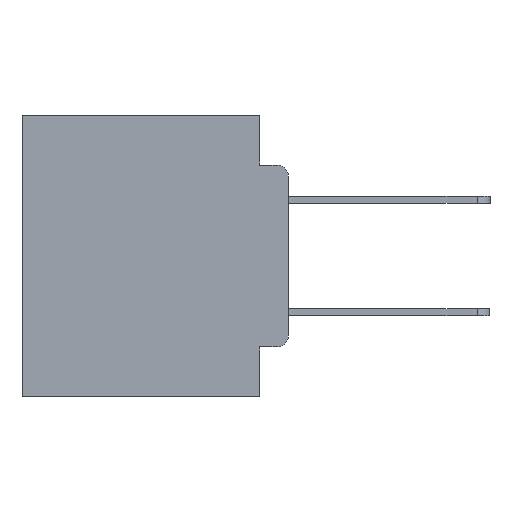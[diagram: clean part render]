
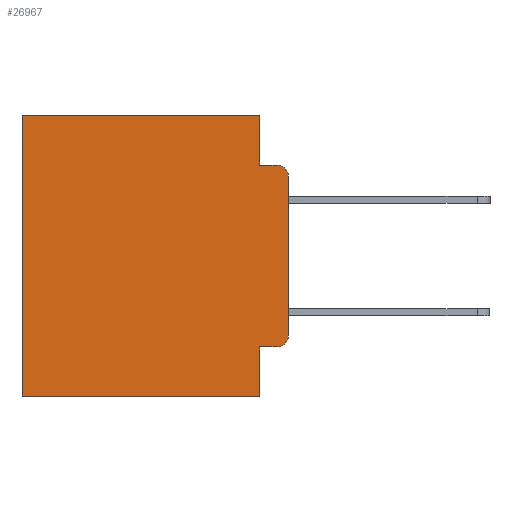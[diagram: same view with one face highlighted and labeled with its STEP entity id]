
A CAD part, left-side view. The second image highlights one B-rep face of the part: STEP entity #26967.
In plain terms, the highlighted planar face has unit normal (-1, 0, 0).
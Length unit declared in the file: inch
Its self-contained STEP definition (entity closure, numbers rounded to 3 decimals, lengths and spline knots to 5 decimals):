
#351 = DIRECTION ( 'NONE',  ( 1., 0., 0. ) ) ;
#569 = VERTEX_POINT ( 'NONE', #1911 ) ;
#1636 = CARTESIAN_POINT ( 'NONE',  ( 0.298, 0., -0.3915 ) ) ;
#1702 = CARTESIAN_POINT ( 'NONE',  ( 0.298, 0.051, -0.0885 ) ) ;
#1837 = EDGE_CURVE ( 'NONE', #15876, #13346, #5750, .T. ) ;
#1911 = CARTESIAN_POINT ( 'NONE',  ( 0.298, 0.02, -0.0885 ) ) ;
#3624 = LINE ( 'NONE', #27789, #20715 ) ;
#3786 = ORIENTED_EDGE ( 'NONE', *, *, #13158, .T. ) ;
#3846 = VECTOR ( 'NONE', #17319, 39.37008 ) ;
#3986 = EDGE_CURVE ( 'NONE', #24738, #13346, #16455, .T. ) ;
#4202 = LINE ( 'NONE', #1702, #21275 ) ;
#4449 = CARTESIAN_POINT ( 'NONE',  ( 0.298, 0.02, -0.4115 ) ) ;
#4802 = AXIS2_PLACEMENT_3D ( 'NONE', #11675, #27195, #13885 ) ;
#4834 = FACE_OUTER_BOUND ( 'NONE', #11723, .T. ) ;
#5104 = VERTEX_POINT ( 'NONE', #20773 ) ;
#5464 = EDGE_CURVE ( 'NONE', #16626, #24738, #8893, .T. ) ;
#5568 = VECTOR ( 'NONE', #9938, 39.37008 ) ;
#5750 = LINE ( 'NONE', #5803, #28702 ) ;
#5803 = CARTESIAN_POINT ( 'NONE',  ( 0.298, 0., 0. ) ) ;
#5854 = CARTESIAN_POINT ( 'NONE',  ( 0.298, 0., -0.1085 ) ) ;
#6951 = CIRCLE ( 'NONE', #4802, 0.02 ) ;
#8451 = EDGE_CURVE ( 'NONE', #16626, #24966, #27492, .T. ) ;
#8736 = VERTEX_POINT ( 'NONE', #20525 ) ;
#8893 = LINE ( 'NONE', #11318, #20067 ) ;
#9236 = DIRECTION ( 'NONE',  ( -1., 0., 0. ) ) ;
#9361 = CARTESIAN_POINT ( 'NONE',  ( 0.298, 0.02, -0.3915 ) ) ;
#9927 = EDGE_CURVE ( 'NONE', #27699, #10752, #15982, .T. ) ;
#9938 = DIRECTION ( 'NONE',  ( 0., 1., 0. ) ) ;
#9998 = DIRECTION ( 'NONE',  ( 0., 1., 0. ) ) ;
#10000 = VECTOR ( 'NONE', #25807, 39.37008 ) ;
#10736 = DIRECTION ( 'NONE',  ( 0., 0., -1. ) ) ;
#10752 = VERTEX_POINT ( 'NONE', #13731 ) ;
#10781 = ORIENTED_EDGE ( 'NONE', *, *, #5464, .T. ) ;
#11318 = CARTESIAN_POINT ( 'NONE',  ( 0.298, 0.051, -0.4115 ) ) ;
#11457 = EDGE_CURVE ( 'NONE', #8736, #5104, #12793, .T. ) ;
#11522 = LINE ( 'NONE', #25519, #5568 ) ;
#11675 = CARTESIAN_POINT ( 'NONE',  ( 0.298, 0.02, -0.1085 ) ) ;
#11723 = EDGE_LOOP ( 'NONE', ( #12921, #28511, #25911, #25845, #3786, #12792, #21637, #26523, #10781, #19932 ) ) ;
#12568 = DIRECTION ( 'NONE',  ( 0., 0., -1. ) ) ;
#12792 = ORIENTED_EDGE ( 'NONE', *, *, #9927, .T. ) ;
#12793 = LINE ( 'NONE', #18281, #23931 ) ;
#12921 = ORIENTED_EDGE ( 'NONE', *, *, #1837, .F. ) ;
#12947 = CARTESIAN_POINT ( 'NONE',  ( 0.298, 0.051, -0.4115 ) ) ;
#13158 = EDGE_CURVE ( 'NONE', #8736, #27699, #3624, .T. ) ;
#13346 = VERTEX_POINT ( 'NONE', #1636 ) ;
#13731 = CARTESIAN_POINT ( 'NONE',  ( 0.298, 0.473, -0.5 ) ) ;
#13855 = CARTESIAN_POINT ( 'NONE',  ( 0.298, 0., 0. ) ) ;
#13885 = DIRECTION ( 'NONE',  ( 0., 0., -1. ) ) ;
#14238 = AXIS2_PLACEMENT_3D ( 'NONE', #9361, #9236, #10736 ) ;
#15164 = DIRECTION ( 'NONE',  ( 0., -1., 0. ) ) ;
#15876 = VERTEX_POINT ( 'NONE', #5854 ) ;
#15982 = LINE ( 'NONE', #19130, #10000 ) ;
#16033 = PLANE ( 'NONE',  #18531 ) ;
#16133 = DIRECTION ( 'NONE',  ( 0., 0., -1. ) ) ;
#16455 = CIRCLE ( 'NONE', #14238, 0.02 ) ;
#16626 = VERTEX_POINT ( 'NONE', #12947 ) ;
#17319 = DIRECTION ( 'NONE',  ( 0., 0., -1. ) ) ;
#18184 = DIRECTION ( 'NONE',  ( 0., 0., -1. ) ) ;
#18281 = CARTESIAN_POINT ( 'NONE',  ( 0.298, 0.051, 0. ) ) ;
#18504 = CARTESIAN_POINT ( 'NONE',  ( 0.298, 0.473, 0. ) ) ;
#18531 = AXIS2_PLACEMENT_3D ( 'NONE', #13855, #351, #16133 ) ;
#18919 = EDGE_CURVE ( 'NONE', #5104, #569, #4202, .T. ) ;
#19130 = CARTESIAN_POINT ( 'NONE',  ( 0.298, 0.473, 0. ) ) ;
#19309 = EDGE_CURVE ( 'NONE', #24966, #10752, #11522, .T. ) ;
#19932 = ORIENTED_EDGE ( 'NONE', *, *, #3986, .T. ) ;
#20067 = VECTOR ( 'NONE', #23649, 39.37008 ) ;
#20417 = EDGE_CURVE ( 'NONE', #15876, #569, #6951, .T. ) ;
#20525 = CARTESIAN_POINT ( 'NONE',  ( 0.298, 0.051, 0. ) ) ;
#20715 = VECTOR ( 'NONE', #9998, 39.37008 ) ;
#20773 = CARTESIAN_POINT ( 'NONE',  ( 0.298, 0.051, -0.0885 ) ) ;
#20799 = CARTESIAN_POINT ( 'NONE',  ( 0.298, 0.051, -0.5 ) ) ;
#21275 = VECTOR ( 'NONE', #15164, 39.37008 ) ;
#21637 = ORIENTED_EDGE ( 'NONE', *, *, #19309, .F. ) ;
#21815 = CARTESIAN_POINT ( 'NONE',  ( 0.298, 0.051, 0. ) ) ;
#23649 = DIRECTION ( 'NONE',  ( 0., -1., 0. ) ) ;
#23931 = VECTOR ( 'NONE', #18184, 39.37008 ) ;
#24738 = VERTEX_POINT ( 'NONE', #4449 ) ;
#24966 = VERTEX_POINT ( 'NONE', #20799 ) ;
#25519 = CARTESIAN_POINT ( 'NONE',  ( 0.298, 0., -0.5 ) ) ;
#25807 = DIRECTION ( 'NONE',  ( 0., 0., -1. ) ) ;
#25845 = ORIENTED_EDGE ( 'NONE', *, *, #11457, .F. ) ;
#25911 = ORIENTED_EDGE ( 'NONE', *, *, #18919, .F. ) ;
#26523 = ORIENTED_EDGE ( 'NONE', *, *, #8451, .F. ) ;
#26967 = ADVANCED_FACE ( 'NONE', ( #4834 ), #16033, .F. ) ;
#27195 = DIRECTION ( 'NONE',  ( -1., 0., 0. ) ) ;
#27492 = LINE ( 'NONE', #21815, #3846 ) ;
#27699 = VERTEX_POINT ( 'NONE', #18504 ) ;
#27789 = CARTESIAN_POINT ( 'NONE',  ( 0.298, 0., 0. ) ) ;
#28511 = ORIENTED_EDGE ( 'NONE', *, *, #20417, .T. ) ;
#28702 = VECTOR ( 'NONE', #12568, 39.37008 ) ;
